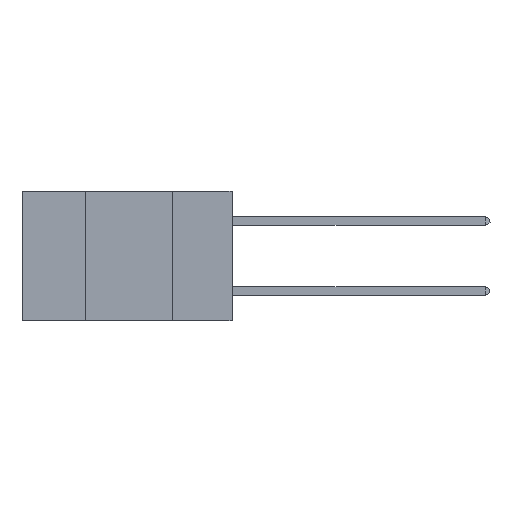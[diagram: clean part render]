
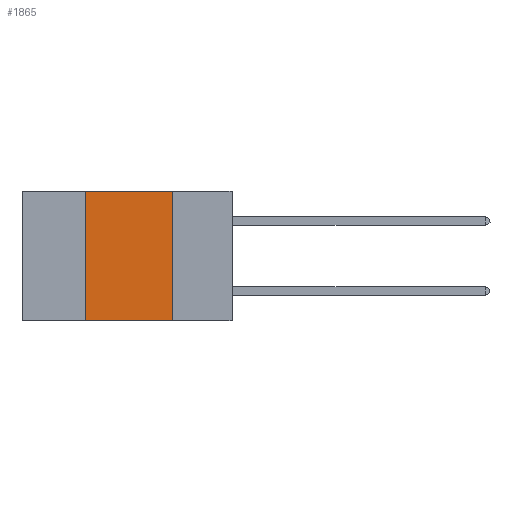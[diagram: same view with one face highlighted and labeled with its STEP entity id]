
A CAD part, left-side view. The second image highlights one B-rep face of the part: STEP entity #1865.
In plain terms, the highlighted planar face has unit normal (-1, 0, 0).
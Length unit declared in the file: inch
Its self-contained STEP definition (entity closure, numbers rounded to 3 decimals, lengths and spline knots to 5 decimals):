
#1001 = ORIENTED_EDGE ( 'NONE', *, *, #12084, .T. ) ;
#1691 = DIRECTION ( 'NONE',  ( 0., -1., 0. ) ) ;
#1792 = CARTESIAN_POINT ( 'NONE',  ( 0., 0.17, 0. ) ) ;
#1865 = ADVANCED_FACE ( 'NONE', ( #3967 ), #5486, .F. ) ;
#1868 = DIRECTION ( 'NONE',  ( 0., 0., -1. ) ) ;
#2413 = EDGE_CURVE ( 'NONE', #18952, #6842, #22833, .T. ) ;
#2709 = CARTESIAN_POINT ( 'NONE',  ( 0., 0.6, -0.37 ) ) ;
#2716 = EDGE_CURVE ( 'NONE', #21272, #18952, #5081, .T. ) ;
#3494 = DIRECTION ( 'NONE',  ( 0., 0., 1. ) ) ;
#3967 = FACE_OUTER_BOUND ( 'NONE', #21966, .T. ) ;
#5081 = LINE ( 'NONE', #5346, #15095 ) ;
#5346 = CARTESIAN_POINT ( 'NONE',  ( 0., 0.42, 0. ) ) ;
#5411 = DIRECTION ( 'NONE',  ( 0., 0., -1. ) ) ;
#5486 = PLANE ( 'NONE',  #18934 ) ;
#5993 = CARTESIAN_POINT ( 'NONE',  ( 0., 0.42, 0. ) ) ;
#6842 = VERTEX_POINT ( 'NONE', #13433 ) ;
#7088 = CARTESIAN_POINT ( 'NONE',  ( 0., 0.6, 0. ) ) ;
#10109 = DIRECTION ( 'NONE',  ( 0., -1., 0. ) ) ;
#11735 = ORIENTED_EDGE ( 'NONE', *, *, #2716, .F. ) ;
#12084 = EDGE_CURVE ( 'NONE', #21272, #15105, #14412, .T. ) ;
#12661 = LINE ( 'NONE', #1792, #16689 ) ;
#13150 = EDGE_CURVE ( 'NONE', #6842, #15105, #12661, .T. ) ;
#13433 = CARTESIAN_POINT ( 'NONE',  ( 0., 0.17, 0. ) ) ;
#14412 = LINE ( 'NONE', #2709, #19564 ) ;
#15095 = VECTOR ( 'NONE', #3494, 39.37008 ) ;
#15105 = VERTEX_POINT ( 'NONE', #20971 ) ;
#15234 = ORIENTED_EDGE ( 'NONE', *, *, #2413, .F. ) ;
#16358 = CARTESIAN_POINT ( 'NONE',  ( 0., 0.42, -0.37 ) ) ;
#16689 = VECTOR ( 'NONE', #1868, 39.37008 ) ;
#18223 = CARTESIAN_POINT ( 'NONE',  ( 0., 0.6, 0. ) ) ;
#18538 = DIRECTION ( 'NONE',  ( 1., 0., 0. ) ) ;
#18934 = AXIS2_PLACEMENT_3D ( 'NONE', #18223, #18538, #5411 ) ;
#18952 = VERTEX_POINT ( 'NONE', #5993 ) ;
#19564 = VECTOR ( 'NONE', #10109, 39.37008 ) ;
#20971 = CARTESIAN_POINT ( 'NONE',  ( 0., 0.17, -0.37 ) ) ;
#21113 = VECTOR ( 'NONE', #1691, 39.37008 ) ;
#21272 = VERTEX_POINT ( 'NONE', #16358 ) ;
#21874 = ORIENTED_EDGE ( 'NONE', *, *, #13150, .F. ) ;
#21966 = EDGE_LOOP ( 'NONE', ( #21874, #15234, #11735, #1001 ) ) ;
#22833 = LINE ( 'NONE', #7088, #21113 ) ;
